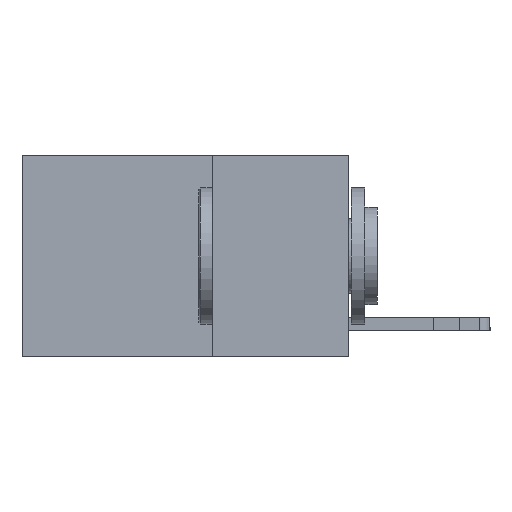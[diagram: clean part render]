
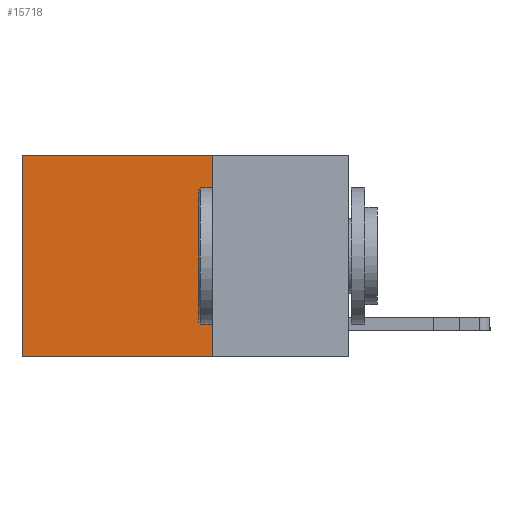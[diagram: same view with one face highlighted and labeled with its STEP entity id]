
A CAD part, left-side view. The second image highlights one B-rep face of the part: STEP entity #15718.
In plain terms, the highlighted planar face has unit normal (-1, 0, 0).
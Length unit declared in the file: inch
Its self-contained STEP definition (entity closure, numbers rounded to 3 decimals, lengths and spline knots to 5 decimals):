
#390 = CARTESIAN_POINT ( 'NONE',  ( 0.2625, 0.6, 0. ) ) ;
#1187 = LINE ( 'NONE', #9564, #9459 ) ;
#1790 = EDGE_CURVE ( 'NONE', #4725, #4923, #6202, .T. ) ;
#1949 = LINE ( 'NONE', #5690, #11623 ) ;
#2061 = DIRECTION ( 'NONE',  ( 0., 1., 0. ) ) ;
#2866 = VECTOR ( 'NONE', #11778, 39.37008 ) ;
#3276 = DIRECTION ( 'NONE',  ( 1., 0., 0. ) ) ;
#3470 = ORIENTED_EDGE ( 'NONE', *, *, #18008, .T. ) ;
#4013 = ORIENTED_EDGE ( 'NONE', *, *, #1790, .F. ) ;
#4615 = CARTESIAN_POINT ( 'NONE',  ( 0.2625, 0.25, 0. ) ) ;
#4638 = PLANE ( 'NONE',  #6035 ) ;
#4725 = VERTEX_POINT ( 'NONE', #11156 ) ;
#4921 = LINE ( 'NONE', #6835, #2866 ) ;
#4923 = VERTEX_POINT ( 'NONE', #10464 ) ;
#5690 = CARTESIAN_POINT ( 'NONE',  ( 0.2625, 0.25, -0.37 ) ) ;
#6035 = AXIS2_PLACEMENT_3D ( 'NONE', #14988, #3276, #6661 ) ;
#6202 = LINE ( 'NONE', #4615, #13400 ) ;
#6661 = DIRECTION ( 'NONE',  ( 0., 0., -1. ) ) ;
#6835 = CARTESIAN_POINT ( 'NONE',  ( 0.2625, 0.25, 0. ) ) ;
#8186 = CARTESIAN_POINT ( 'NONE',  ( 0.2625, 0.6, -0.37 ) ) ;
#8611 = EDGE_CURVE ( 'NONE', #19814, #19150, #1187, .T. ) ;
#8901 = FACE_OUTER_BOUND ( 'NONE', #14829, .T. ) ;
#9145 = ORIENTED_EDGE ( 'NONE', *, *, #9308, .F. ) ;
#9308 = EDGE_CURVE ( 'NONE', #4923, #19150, #1949, .T. ) ;
#9459 = VECTOR ( 'NONE', #16430, 39.37008 ) ;
#9564 = CARTESIAN_POINT ( 'NONE',  ( 0.2625, 0.6, 0. ) ) ;
#10464 = CARTESIAN_POINT ( 'NONE',  ( 0.2625, 0.25, -0.37 ) ) ;
#11156 = CARTESIAN_POINT ( 'NONE',  ( 0.2625, 0.25, 0. ) ) ;
#11623 = VECTOR ( 'NONE', #2061, 39.37008 ) ;
#11778 = DIRECTION ( 'NONE',  ( 0., 1., 0. ) ) ;
#13400 = VECTOR ( 'NONE', #16896, 39.37008 ) ;
#14829 = EDGE_LOOP ( 'NONE', ( #18075, #9145, #4013, #3470 ) ) ;
#14988 = CARTESIAN_POINT ( 'NONE',  ( 0.2625, 0.25, 0. ) ) ;
#15718 = ADVANCED_FACE ( 'NONE', ( #8901 ), #4638, .F. ) ;
#16430 = DIRECTION ( 'NONE',  ( 0., 0., -1. ) ) ;
#16896 = DIRECTION ( 'NONE',  ( 0., 0., -1. ) ) ;
#18008 = EDGE_CURVE ( 'NONE', #4725, #19814, #4921, .T. ) ;
#18075 = ORIENTED_EDGE ( 'NONE', *, *, #8611, .T. ) ;
#19150 = VERTEX_POINT ( 'NONE', #8186 ) ;
#19814 = VERTEX_POINT ( 'NONE', #390 ) ;
